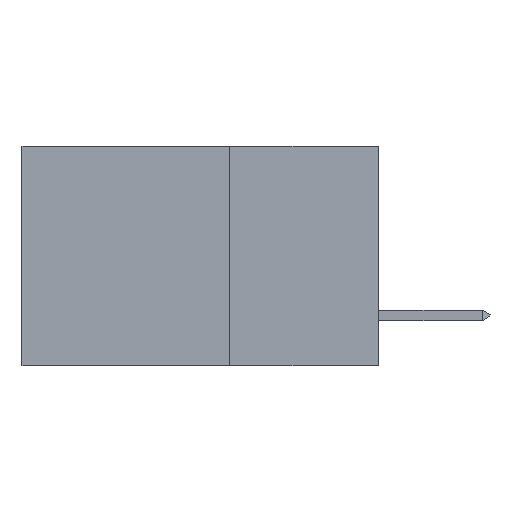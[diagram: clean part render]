
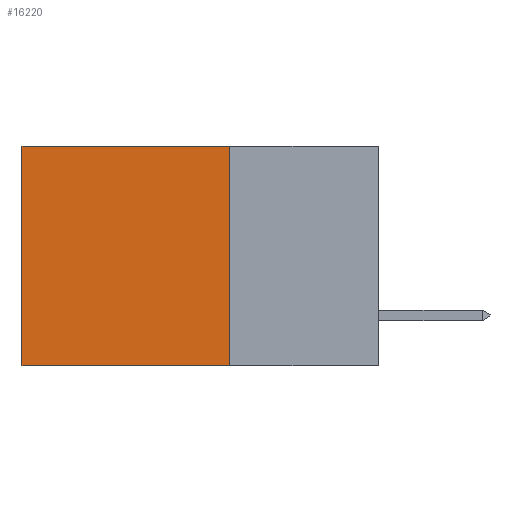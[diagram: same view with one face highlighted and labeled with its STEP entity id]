
A CAD part, left-side view. The second image highlights one B-rep face of the part: STEP entity #16220.
In plain terms, the highlighted planar face has unit normal (-1, 0, 0).
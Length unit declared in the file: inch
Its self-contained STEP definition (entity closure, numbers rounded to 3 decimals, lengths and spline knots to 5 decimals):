
#2035 = CARTESIAN_POINT ( 'NONE',  ( 0.298, 0.6, -0.37 ) ) ;
#2860 = AXIS2_PLACEMENT_3D ( 'NONE', #8253, #15611, #22834 ) ;
#3001 = VECTOR ( 'NONE', #31922, 39.37008 ) ;
#3096 = DIRECTION ( 'NONE',  ( 0., 1., 0. ) ) ;
#3190 = PLANE ( 'NONE',  #2860 ) ;
#6247 = CARTESIAN_POINT ( 'NONE',  ( 0.298, 0.6, 0. ) ) ;
#6925 = EDGE_CURVE ( 'NONE', #26483, #18976, #29754, .T. ) ;
#8253 = CARTESIAN_POINT ( 'NONE',  ( 0.298, 0.25, 0. ) ) ;
#8952 = VECTOR ( 'NONE', #3096, 39.37008 ) ;
#11364 = CARTESIAN_POINT ( 'NONE',  ( 0.298, 0.25, -0.37 ) ) ;
#13703 = EDGE_CURVE ( 'NONE', #30226, #28160, #15392, .T. ) ;
#13799 = LINE ( 'NONE', #31536, #22278 ) ;
#15392 = LINE ( 'NONE', #16386, #23494 ) ;
#15611 = DIRECTION ( 'NONE',  ( 1., 0., 0. ) ) ;
#16220 = ADVANCED_FACE ( 'NONE', ( #27520 ), #3190, .F. ) ;
#16386 = CARTESIAN_POINT ( 'NONE',  ( 0.298, 0.25, 0. ) ) ;
#18976 = VERTEX_POINT ( 'NONE', #2035 ) ;
#20466 = ORIENTED_EDGE ( 'NONE', *, *, #6925, .F. ) ;
#21091 = ORIENTED_EDGE ( 'NONE', *, *, #29827, .T. ) ;
#21351 = DIRECTION ( 'NONE',  ( 0., 1., 0. ) ) ;
#22278 = VECTOR ( 'NONE', #24141, 39.37008 ) ;
#22834 = DIRECTION ( 'NONE',  ( 0., 0., -1. ) ) ;
#23494 = VECTOR ( 'NONE', #21351, 39.37008 ) ;
#23658 = ORIENTED_EDGE ( 'NONE', *, *, #13703, .T. ) ;
#24141 = DIRECTION ( 'NONE',  ( 0., 0., -1. ) ) ;
#24279 = EDGE_CURVE ( 'NONE', #30226, #26483, #27662, .T. ) ;
#26023 = CARTESIAN_POINT ( 'NONE',  ( 0.298, 0.25, 0. ) ) ;
#26268 = EDGE_LOOP ( 'NONE', ( #21091, #20466, #26785, #23658 ) ) ;
#26483 = VERTEX_POINT ( 'NONE', #11364 ) ;
#26785 = ORIENTED_EDGE ( 'NONE', *, *, #24279, .F. ) ;
#27520 = FACE_OUTER_BOUND ( 'NONE', #26268, .T. ) ;
#27662 = LINE ( 'NONE', #26023, #3001 ) ;
#27859 = CARTESIAN_POINT ( 'NONE',  ( 0.298, 0.25, -0.37 ) ) ;
#28160 = VERTEX_POINT ( 'NONE', #6247 ) ;
#29754 = LINE ( 'NONE', #27859, #8952 ) ;
#29827 = EDGE_CURVE ( 'NONE', #28160, #18976, #13799, .T. ) ;
#30226 = VERTEX_POINT ( 'NONE', #30519 ) ;
#30519 = CARTESIAN_POINT ( 'NONE',  ( 0.298, 0.25, 0. ) ) ;
#31536 = CARTESIAN_POINT ( 'NONE',  ( 0.298, 0.6, 0. ) ) ;
#31922 = DIRECTION ( 'NONE',  ( 0., 0., -1. ) ) ;
